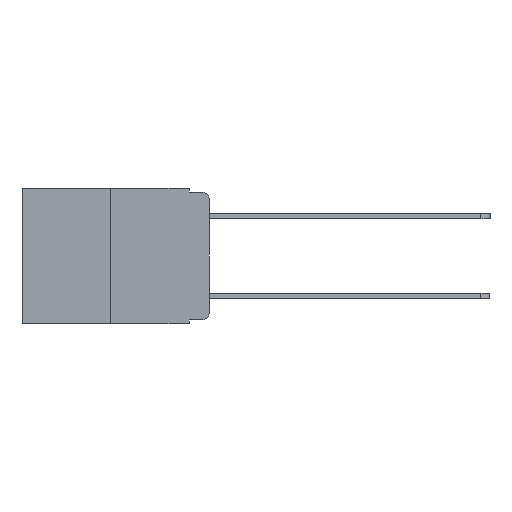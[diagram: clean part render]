
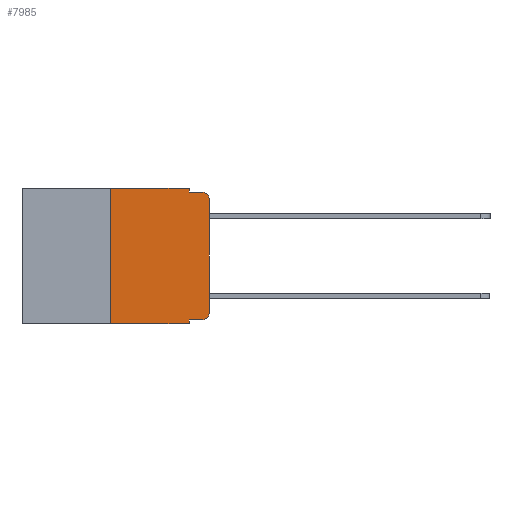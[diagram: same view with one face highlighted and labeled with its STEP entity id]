
A CAD part, left-side view. The second image highlights one B-rep face of the part: STEP entity #7985.
In plain terms, the highlighted planar face has unit normal (-1, 0, 0).
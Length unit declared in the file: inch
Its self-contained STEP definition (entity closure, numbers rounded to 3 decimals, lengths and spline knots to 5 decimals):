
#83 = ORIENTED_EDGE ( 'NONE', *, *, #6790, .F. ) ;
#323 = DIRECTION ( 'NONE',  ( 1., 0., 0. ) ) ;
#454 = VERTEX_POINT ( 'NONE', #10617 ) ;
#481 = LINE ( 'NONE', #1605, #11892 ) ;
#970 = CARTESIAN_POINT ( 'NONE',  ( 0., 0.02, -0.333 ) ) ;
#1096 = ORIENTED_EDGE ( 'NONE', *, *, #6813, .T. ) ;
#1322 = AXIS2_PLACEMENT_3D ( 'NONE', #9474, #2784, #10407 ) ;
#1350 = VECTOR ( 'NONE', #7455, 39.37008 ) ;
#1382 = CARTESIAN_POINT ( 'NONE',  ( 0., 0.25, -0.343 ) ) ;
#1413 = ORIENTED_EDGE ( 'NONE', *, *, #6550, .T. ) ;
#1605 = CARTESIAN_POINT ( 'NONE',  ( 0., 0.051, 0. ) ) ;
#2784 = DIRECTION ( 'NONE',  ( -1., 0., 0. ) ) ;
#3321 = LINE ( 'NONE', #12015, #5739 ) ;
#3611 = CARTESIAN_POINT ( 'NONE',  ( 0., 0.051, -0.01 ) ) ;
#3666 = CIRCLE ( 'NONE', #1322, 0.02 ) ;
#3850 = LINE ( 'NONE', #5245, #6619 ) ;
#3908 = CARTESIAN_POINT ( 'NONE',  ( 0., 0.051, 0. ) ) ;
#4113 = CARTESIAN_POINT ( 'NONE',  ( 0., 0.02, -0.313 ) ) ;
#4231 = LINE ( 'NONE', #8556, #12174 ) ;
#4621 = LINE ( 'NONE', #11354, #9952 ) ;
#4675 = ORIENTED_EDGE ( 'NONE', *, *, #6807, .F. ) ;
#4713 = VERTEX_POINT ( 'NONE', #11451 ) ;
#4722 = AXIS2_PLACEMENT_3D ( 'NONE', #9544, #323, #8641 ) ;
#4970 = LINE ( 'NONE', #12269, #10234 ) ;
#5093 = ORIENTED_EDGE ( 'NONE', *, *, #6816, .T. ) ;
#5245 = CARTESIAN_POINT ( 'NONE',  ( 0., 0.051, -0.333 ) ) ;
#5288 = DIRECTION ( 'NONE',  ( 0., 0., -1. ) ) ;
#5373 = AXIS2_PLACEMENT_3D ( 'NONE', #4113, #11435, #5288 ) ;
#5739 = VECTOR ( 'NONE', #12916, 39.37008 ) ;
#5754 = EDGE_LOOP ( 'NONE', ( #11447, #11017, #9845, #10733, #11026, #83, #1413, #4675, #1096, #5093 ) ) ;
#6124 = EDGE_CURVE ( 'NONE', #4713, #8710, #3321, .T. ) ;
#6320 = VERTEX_POINT ( 'NONE', #10503 ) ;
#6420 = DIRECTION ( 'NONE',  ( 0., 0., -1. ) ) ;
#6550 = EDGE_CURVE ( 'NONE', #6716, #9455, #9099, .T. ) ;
#6619 = VECTOR ( 'NONE', #8601, 39.37008 ) ;
#6716 = VERTEX_POINT ( 'NONE', #1382 ) ;
#6750 = EDGE_CURVE ( 'NONE', #8105, #11738, #4970, .T. ) ;
#6766 = EDGE_CURVE ( 'NONE', #11738, #454, #3666, .T. ) ;
#6768 = EDGE_CURVE ( 'NONE', #8250, #454, #12744, .T. ) ;
#6771 = EDGE_CURVE ( 'NONE', #8710, #8250, #4621, .T. ) ;
#6790 = EDGE_CURVE ( 'NONE', #6716, #4713, #4231, .T. ) ;
#6807 = EDGE_CURVE ( 'NONE', #6320, #9455, #481, .T. ) ;
#6813 = EDGE_CURVE ( 'NONE', #6320, #9767, #3850, .T. ) ;
#6816 = EDGE_CURVE ( 'NONE', #9767, #8105, #9377, .T. ) ;
#7455 = DIRECTION ( 'NONE',  ( 0., -1., 0. ) ) ;
#7856 = CARTESIAN_POINT ( 'NONE',  ( 0., 0., -0.313 ) ) ;
#7985 = ADVANCED_FACE ( 'NONE', ( #8116 ), #13270, .F. ) ;
#8105 = VERTEX_POINT ( 'NONE', #7856 ) ;
#8108 = CARTESIAN_POINT ( 'NONE',  ( 0., 0.473, -0.343 ) ) ;
#8116 = FACE_OUTER_BOUND ( 'NONE', #5754, .T. ) ;
#8250 = VERTEX_POINT ( 'NONE', #3611 ) ;
#8556 = CARTESIAN_POINT ( 'NONE',  ( 0., 0.25, 0. ) ) ;
#8601 = DIRECTION ( 'NONE',  ( 0., -1., 0. ) ) ;
#8641 = DIRECTION ( 'NONE',  ( 0., 0., -1. ) ) ;
#8710 = VERTEX_POINT ( 'NONE', #3908 ) ;
#9099 = LINE ( 'NONE', #8108, #13704 ) ;
#9118 = DIRECTION ( 'NONE',  ( 0., -1., 0. ) ) ;
#9377 = CIRCLE ( 'NONE', #5373, 0.02 ) ;
#9430 = CARTESIAN_POINT ( 'NONE',  ( 0., 0.051, -0.01 ) ) ;
#9455 = VERTEX_POINT ( 'NONE', #12633 ) ;
#9474 = CARTESIAN_POINT ( 'NONE',  ( 0., 0.02, -0.03 ) ) ;
#9513 = DIRECTION ( 'NONE',  ( 0., 0., 1. ) ) ;
#9544 = CARTESIAN_POINT ( 'NONE',  ( 0., 0.473, 0. ) ) ;
#9767 = VERTEX_POINT ( 'NONE', #970 ) ;
#9845 = ORIENTED_EDGE ( 'NONE', *, *, #6768, .F. ) ;
#9952 = VECTOR ( 'NONE', #12310, 39.37008 ) ;
#10234 = VECTOR ( 'NONE', #13164, 39.37008 ) ;
#10407 = DIRECTION ( 'NONE',  ( 0., 0., -1. ) ) ;
#10503 = CARTESIAN_POINT ( 'NONE',  ( 0., 0.051, -0.333 ) ) ;
#10617 = CARTESIAN_POINT ( 'NONE',  ( 0., 0.02, -0.01 ) ) ;
#10733 = ORIENTED_EDGE ( 'NONE', *, *, #6771, .F. ) ;
#11017 = ORIENTED_EDGE ( 'NONE', *, *, #6766, .T. ) ;
#11026 = ORIENTED_EDGE ( 'NONE', *, *, #6124, .F. ) ;
#11354 = CARTESIAN_POINT ( 'NONE',  ( 0., 0.051, 0. ) ) ;
#11435 = DIRECTION ( 'NONE',  ( -1., 0., 0. ) ) ;
#11447 = ORIENTED_EDGE ( 'NONE', *, *, #6750, .T. ) ;
#11451 = CARTESIAN_POINT ( 'NONE',  ( 0., 0.25, 0. ) ) ;
#11738 = VERTEX_POINT ( 'NONE', #13273 ) ;
#11892 = VECTOR ( 'NONE', #6420, 39.37008 ) ;
#12015 = CARTESIAN_POINT ( 'NONE',  ( 0., 0.473, 0. ) ) ;
#12174 = VECTOR ( 'NONE', #9513, 39.37008 ) ;
#12269 = CARTESIAN_POINT ( 'NONE',  ( 0., 0., 0. ) ) ;
#12310 = DIRECTION ( 'NONE',  ( 0., 0., -1. ) ) ;
#12633 = CARTESIAN_POINT ( 'NONE',  ( 0., 0.051, -0.343 ) ) ;
#12744 = LINE ( 'NONE', #9430, #1350 ) ;
#12916 = DIRECTION ( 'NONE',  ( 0., -1., 0. ) ) ;
#13164 = DIRECTION ( 'NONE',  ( 0., 0., 1. ) ) ;
#13270 = PLANE ( 'NONE',  #4722 ) ;
#13273 = CARTESIAN_POINT ( 'NONE',  ( 0., 0., -0.03 ) ) ;
#13704 = VECTOR ( 'NONE', #9118, 39.37008 ) ;
